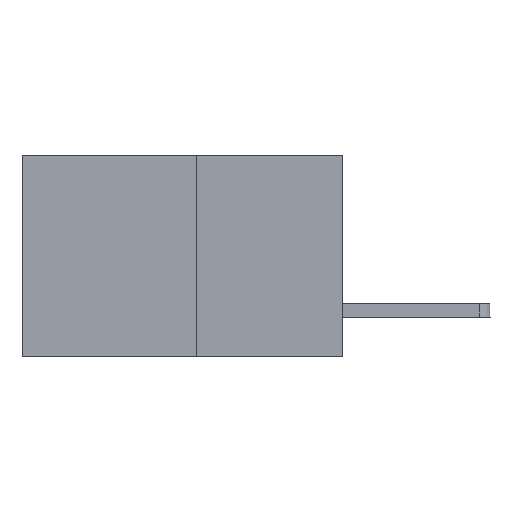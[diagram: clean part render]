
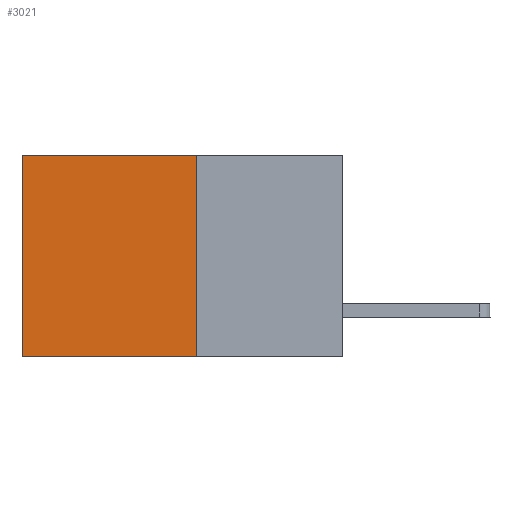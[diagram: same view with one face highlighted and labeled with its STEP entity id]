
A CAD part, left-side view. The second image highlights one B-rep face of the part: STEP entity #3021.
In plain terms, the highlighted planar face has unit normal (-1, 0, 0).
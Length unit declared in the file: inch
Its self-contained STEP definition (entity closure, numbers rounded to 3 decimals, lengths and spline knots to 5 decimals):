
#7 = CARTESIAN_POINT ( 'NONE',  ( 0.277, 0.27, 0. ) ) ;
#78 = AXIS2_PLACEMENT_3D ( 'NONE', #6001, #1652, #367 ) ;
#226 = VECTOR ( 'NONE', #1811, 39.37008 ) ;
#367 = DIRECTION ( 'NONE',  ( 0., 0., -1. ) ) ;
#613 = VECTOR ( 'NONE', #4065, 39.37008 ) ;
#1097 = CARTESIAN_POINT ( 'NONE',  ( 0.277, 0.59, -0.37 ) ) ;
#1118 = CARTESIAN_POINT ( 'NONE',  ( 0.277, 0.27, -0.37 ) ) ;
#1135 = LINE ( 'NONE', #1097, #226 ) ;
#1233 = ORIENTED_EDGE ( 'NONE', *, *, #2254, .T. ) ;
#1652 = DIRECTION ( 'NONE',  ( 1., 0., 0. ) ) ;
#1766 = DIRECTION ( 'NONE',  ( 0., 1., 0. ) ) ;
#1811 = DIRECTION ( 'NONE',  ( 0., 0., -1. ) ) ;
#2254 = EDGE_CURVE ( 'NONE', #3659, #6201, #7503, .T. ) ;
#2410 = VERTEX_POINT ( 'NONE', #4426 ) ;
#2481 = CARTESIAN_POINT ( 'NONE',  ( 0.277, 0.27, 0. ) ) ;
#3021 = ADVANCED_FACE ( 'NONE', ( #5454 ), #6085, .F. ) ;
#3574 = EDGE_CURVE ( 'NONE', #6201, #2410, #1135, .T. ) ;
#3600 = ORIENTED_EDGE ( 'NONE', *, *, #8141, .F. ) ;
#3659 = VERTEX_POINT ( 'NONE', #7 ) ;
#3808 = EDGE_CURVE ( 'NONE', #6508, #2410, #5353, .T. ) ;
#4065 = DIRECTION ( 'NONE',  ( 0., 0., -1. ) ) ;
#4426 = CARTESIAN_POINT ( 'NONE',  ( 0.277, 0.59, -0.37 ) ) ;
#4795 = DIRECTION ( 'NONE',  ( 0., 1., 0. ) ) ;
#5151 = CARTESIAN_POINT ( 'NONE',  ( 0.277, 0.59, 0. ) ) ;
#5353 = LINE ( 'NONE', #6023, #7843 ) ;
#5454 = FACE_OUTER_BOUND ( 'NONE', #5560, .T. ) ;
#5560 = EDGE_LOOP ( 'NONE', ( #5862, #7588, #3600, #1233 ) ) ;
#5862 = ORIENTED_EDGE ( 'NONE', *, *, #3574, .T. ) ;
#6001 = CARTESIAN_POINT ( 'NONE',  ( 0.277, 0.27, -0.37 ) ) ;
#6023 = CARTESIAN_POINT ( 'NONE',  ( 0.277, 0.27, -0.37 ) ) ;
#6085 = PLANE ( 'NONE',  #78 ) ;
#6201 = VERTEX_POINT ( 'NONE', #5151 ) ;
#6508 = VERTEX_POINT ( 'NONE', #1118 ) ;
#6852 = VECTOR ( 'NONE', #1766, 39.37008 ) ;
#7293 = CARTESIAN_POINT ( 'NONE',  ( 0.277, 0.27, -0.37 ) ) ;
#7503 = LINE ( 'NONE', #2481, #6852 ) ;
#7510 = LINE ( 'NONE', #7293, #613 ) ;
#7588 = ORIENTED_EDGE ( 'NONE', *, *, #3808, .F. ) ;
#7843 = VECTOR ( 'NONE', #4795, 39.37008 ) ;
#8141 = EDGE_CURVE ( 'NONE', #3659, #6508, #7510, .T. ) ;
